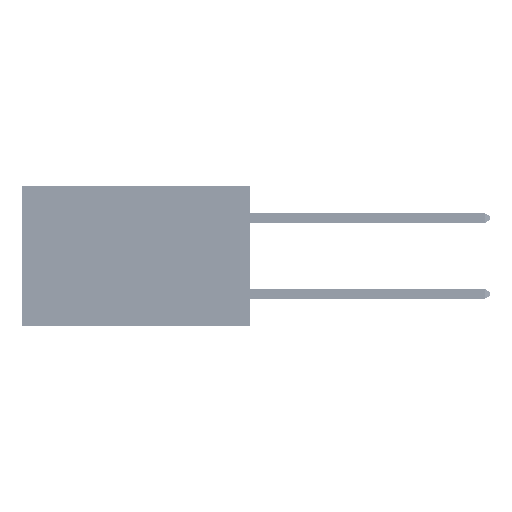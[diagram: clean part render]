
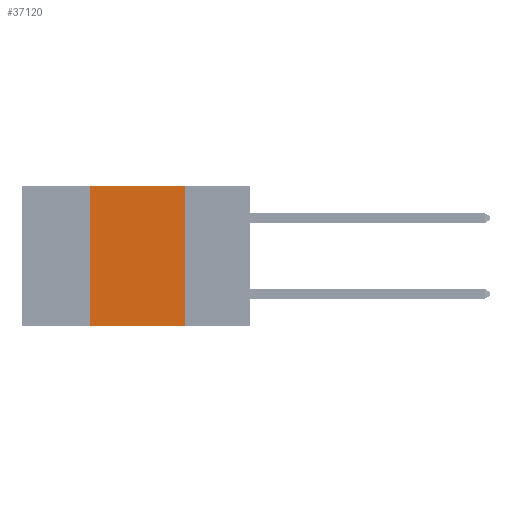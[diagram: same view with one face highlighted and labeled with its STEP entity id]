
A CAD part, left-side view. The second image highlights one B-rep face of the part: STEP entity #37120.
In plain terms, the highlighted planar face has unit normal (-1, 0, 0).
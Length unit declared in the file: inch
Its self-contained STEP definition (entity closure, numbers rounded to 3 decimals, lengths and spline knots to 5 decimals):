
#362 = VERTEX_POINT ( 'NONE', #48614 ) ;
#1557 = FACE_OUTER_BOUND ( 'NONE', #26137, .T. ) ;
#1881 = VERTEX_POINT ( 'NONE', #18112 ) ;
#2039 = CARTESIAN_POINT ( 'NONE',  ( 0., 0.42, 0. ) ) ;
#2360 = PLANE ( 'NONE',  #18231 ) ;
#3939 = DIRECTION ( 'NONE',  ( 0., -1., 0. ) ) ;
#4359 = DIRECTION ( 'NONE',  ( 0., 0., -1. ) ) ;
#6638 = ORIENTED_EDGE ( 'NONE', *, *, #38368, .F. ) ;
#6651 = CARTESIAN_POINT ( 'NONE',  ( 0., 0.6, 0. ) ) ;
#10376 = DIRECTION ( 'NONE',  ( 0., 0., -1. ) ) ;
#11776 = ORIENTED_EDGE ( 'NONE', *, *, #11947, .F. ) ;
#11947 = EDGE_CURVE ( 'NONE', #362, #1881, #14466, .T. ) ;
#14466 = LINE ( 'NONE', #20554, #18274 ) ;
#14901 = VECTOR ( 'NONE', #36175, 39.37008 ) ;
#18112 = CARTESIAN_POINT ( 'NONE',  ( 0., 0.17, -0.37 ) ) ;
#18231 = AXIS2_PLACEMENT_3D ( 'NONE', #6651, #34502, #10376 ) ;
#18274 = VECTOR ( 'NONE', #4359, 39.37008 ) ;
#19673 = VECTOR ( 'NONE', #3939, 39.37008 ) ;
#20554 = CARTESIAN_POINT ( 'NONE',  ( 0., 0.17, 0. ) ) ;
#22805 = CARTESIAN_POINT ( 'NONE',  ( 0., 0.42, 0. ) ) ;
#23678 = EDGE_CURVE ( 'NONE', #47468, #362, #41514, .T. ) ;
#26137 = EDGE_LOOP ( 'NONE', ( #11776, #28315, #6638, #45008 ) ) ;
#28315 = ORIENTED_EDGE ( 'NONE', *, *, #23678, .F. ) ;
#28543 = CARTESIAN_POINT ( 'NONE',  ( 0., 0.6, 0. ) ) ;
#32185 = CARTESIAN_POINT ( 'NONE',  ( 0., 0.6, -0.37 ) ) ;
#34502 = DIRECTION ( 'NONE',  ( 1., 0., 0. ) ) ;
#35365 = DIRECTION ( 'NONE',  ( 0., 0., 1. ) ) ;
#36175 = DIRECTION ( 'NONE',  ( 0., -1., 0. ) ) ;
#36332 = VECTOR ( 'NONE', #35365, 39.37008 ) ;
#37120 = ADVANCED_FACE ( 'NONE', ( #1557 ), #2360, .F. ) ;
#38368 = EDGE_CURVE ( 'NONE', #38753, #47468, #47113, .T. ) ;
#38753 = VERTEX_POINT ( 'NONE', #48611 ) ;
#40275 = EDGE_CURVE ( 'NONE', #38753, #1881, #41820, .T. ) ;
#41514 = LINE ( 'NONE', #28543, #14901 ) ;
#41820 = LINE ( 'NONE', #32185, #19673 ) ;
#45008 = ORIENTED_EDGE ( 'NONE', *, *, #40275, .T. ) ;
#47113 = LINE ( 'NONE', #22805, #36332 ) ;
#47468 = VERTEX_POINT ( 'NONE', #2039 ) ;
#48611 = CARTESIAN_POINT ( 'NONE',  ( 0., 0.42, -0.37 ) ) ;
#48614 = CARTESIAN_POINT ( 'NONE',  ( 0., 0.17, 0. ) ) ;
